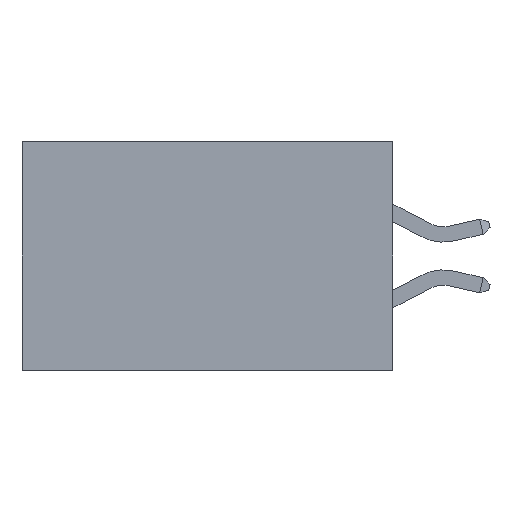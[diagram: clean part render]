
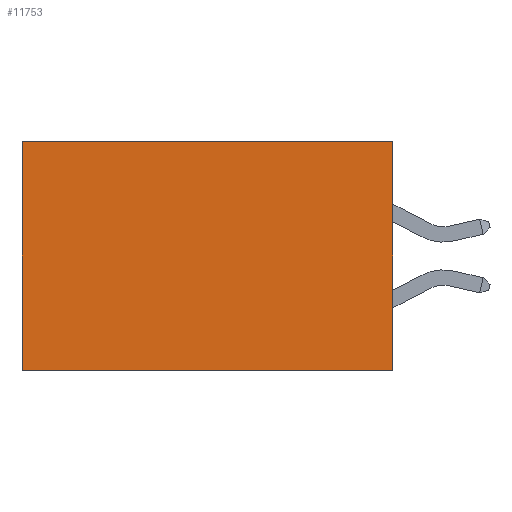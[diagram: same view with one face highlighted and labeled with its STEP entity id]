
A CAD part, left-side view. The second image highlights one B-rep face of the part: STEP entity #11753.
In plain terms, the highlighted planar face has unit normal (-1, 0, 0).
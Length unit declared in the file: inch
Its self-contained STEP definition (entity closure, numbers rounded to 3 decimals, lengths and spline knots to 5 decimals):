
#107 = EDGE_CURVE ( 'NONE', #9568, #3414, #29447, .T. ) ;
#484 = VECTOR ( 'NONE', #21551, 39.37008 ) ;
#880 = DIRECTION ( 'NONE',  ( 0., 0., -1. ) ) ;
#2120 = CARTESIAN_POINT ( 'NONE',  ( 0.2875, 0., 0. ) ) ;
#2699 = CARTESIAN_POINT ( 'NONE',  ( 0.2875, 0., 0. ) ) ;
#3414 = VERTEX_POINT ( 'NONE', #22919 ) ;
#5005 = EDGE_CURVE ( 'NONE', #9568, #27034, #17888, .T. ) ;
#8030 = LINE ( 'NONE', #16344, #22794 ) ;
#9141 = EDGE_CURVE ( 'NONE', #27034, #9533, #8030, .T. ) ;
#9533 = VERTEX_POINT ( 'NONE', #39579 ) ;
#9568 = VERTEX_POINT ( 'NONE', #2699 ) ;
#11753 = ADVANCED_FACE ( 'NONE', ( #14348 ), #13239, .F. ) ;
#13239 = PLANE ( 'NONE',  #25408 ) ;
#13894 = DIRECTION ( 'NONE',  ( 0., 0., -1. ) ) ;
#14348 = FACE_OUTER_BOUND ( 'NONE', #34105, .T. ) ;
#16303 = CARTESIAN_POINT ( 'NONE',  ( 0.2875, 0., 0. ) ) ;
#16344 = CARTESIAN_POINT ( 'NONE',  ( 0.2875, 0., -0.37 ) ) ;
#17888 = LINE ( 'NONE', #30755, #484 ) ;
#19401 = DIRECTION ( 'NONE',  ( 1., 0., 0. ) ) ;
#19441 = DIRECTION ( 'NONE',  ( 0., 1., 0. ) ) ;
#21551 = DIRECTION ( 'NONE',  ( 0., 0., -1. ) ) ;
#22336 = ORIENTED_EDGE ( 'NONE', *, *, #107, .T. ) ;
#22694 = ORIENTED_EDGE ( 'NONE', *, *, #32872, .T. ) ;
#22794 = VECTOR ( 'NONE', #19441, 39.37008 ) ;
#22919 = CARTESIAN_POINT ( 'NONE',  ( 0.2875, 0.6, 0. ) ) ;
#23761 = ORIENTED_EDGE ( 'NONE', *, *, #5005, .F. ) ;
#25408 = AXIS2_PLACEMENT_3D ( 'NONE', #16303, #19401, #880 ) ;
#26206 = VECTOR ( 'NONE', #13894, 39.37008 ) ;
#27034 = VERTEX_POINT ( 'NONE', #35905 ) ;
#27654 = ORIENTED_EDGE ( 'NONE', *, *, #9141, .F. ) ;
#29109 = DIRECTION ( 'NONE',  ( 0., 1., 0. ) ) ;
#29447 = LINE ( 'NONE', #2120, #35679 ) ;
#30755 = CARTESIAN_POINT ( 'NONE',  ( 0.2875, 0., 0. ) ) ;
#32872 = EDGE_CURVE ( 'NONE', #3414, #9533, #34350, .T. ) ;
#34105 = EDGE_LOOP ( 'NONE', ( #22694, #27654, #23761, #22336 ) ) ;
#34350 = LINE ( 'NONE', #35492, #26206 ) ;
#35492 = CARTESIAN_POINT ( 'NONE',  ( 0.2875, 0.6, 0. ) ) ;
#35679 = VECTOR ( 'NONE', #29109, 39.37008 ) ;
#35905 = CARTESIAN_POINT ( 'NONE',  ( 0.2875, 0., -0.37 ) ) ;
#39579 = CARTESIAN_POINT ( 'NONE',  ( 0.2875, 0.6, -0.37 ) ) ;
